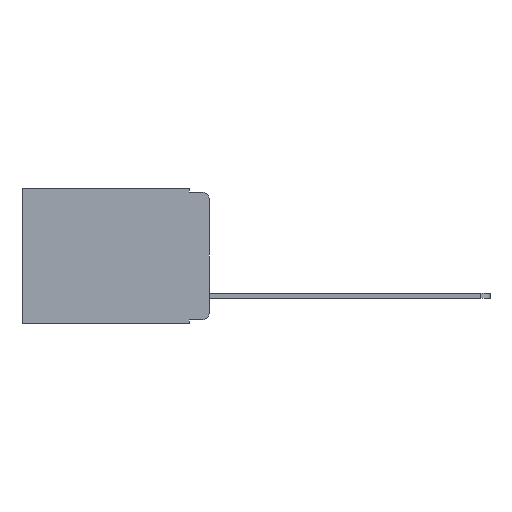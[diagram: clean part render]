
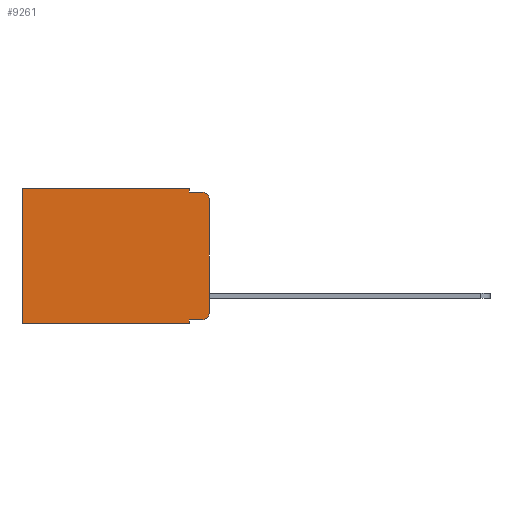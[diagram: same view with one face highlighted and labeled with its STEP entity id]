
A CAD part, left-side view. The second image highlights one B-rep face of the part: STEP entity #9261.
In plain terms, the highlighted planar face has unit normal (-1, 0, 0).
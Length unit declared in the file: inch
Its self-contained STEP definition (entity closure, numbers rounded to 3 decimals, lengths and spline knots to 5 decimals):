
#23 = VERTEX_POINT ( 'NONE', #14910 ) ;
#383 = VERTEX_POINT ( 'NONE', #16294 ) ;
#658 = VERTEX_POINT ( 'NONE', #15442 ) ;
#695 = EDGE_CURVE ( 'NONE', #15312, #2778, #7345, .T. ) ;
#776 = VERTEX_POINT ( 'NONE', #18592 ) ;
#1225 = DIRECTION ( 'NONE',  ( 0., -1., 0. ) ) ;
#1609 = CARTESIAN_POINT ( 'NONE',  ( 0.298, 0., -0.343 ) ) ;
#1758 = PLANE ( 'NONE',  #10505 ) ;
#1880 = EDGE_CURVE ( 'NONE', #15836, #3848, #2449, .T. ) ;
#2449 = LINE ( 'NONE', #13862, #15797 ) ;
#2712 = DIRECTION ( 'NONE',  ( 0., 1., 0. ) ) ;
#2778 = VERTEX_POINT ( 'NONE', #19529 ) ;
#3136 = DIRECTION ( 'NONE',  ( -1., 0., 0. ) ) ;
#3154 = CIRCLE ( 'NONE', #19456, 0.02 ) ;
#3315 = VECTOR ( 'NONE', #5081, 39.37008 ) ;
#3368 = VECTOR ( 'NONE', #15192, 39.37008 ) ;
#3510 = CARTESIAN_POINT ( 'NONE',  ( 0.298, 0., 0. ) ) ;
#3606 = CARTESIAN_POINT ( 'NONE',  ( 0.298, 0.02, -0.03 ) ) ;
#3813 = ORIENTED_EDGE ( 'NONE', *, *, #19001, .F. ) ;
#3848 = VERTEX_POINT ( 'NONE', #4639 ) ;
#3917 = LINE ( 'NONE', #19953, #3368 ) ;
#4080 = ORIENTED_EDGE ( 'NONE', *, *, #5950, .F. ) ;
#4222 = EDGE_CURVE ( 'NONE', #15836, #23, #12175, .T. ) ;
#4639 = CARTESIAN_POINT ( 'NONE',  ( 0.298, 0.02, -0.333 ) ) ;
#4888 = CARTESIAN_POINT ( 'NONE',  ( 0.298, 0.051, 0. ) ) ;
#4897 = CARTESIAN_POINT ( 'NONE',  ( 0.298, 0.051, 0. ) ) ;
#5081 = DIRECTION ( 'NONE',  ( 0., 0., -1. ) ) ;
#5204 = VERTEX_POINT ( 'NONE', #5229 ) ;
#5229 = CARTESIAN_POINT ( 'NONE',  ( 0.298, 0.473, -0.343 ) ) ;
#5275 = DIRECTION ( 'NONE',  ( 1., 0., 0. ) ) ;
#5374 = DIRECTION ( 'NONE',  ( 0., 0., -1. ) ) ;
#5455 = ORIENTED_EDGE ( 'NONE', *, *, #15792, .F. ) ;
#5950 = EDGE_CURVE ( 'NONE', #23, #5204, #6473, .T. ) ;
#5974 = ORIENTED_EDGE ( 'NONE', *, *, #7655, .T. ) ;
#6473 = LINE ( 'NONE', #1609, #18988 ) ;
#6525 = ORIENTED_EDGE ( 'NONE', *, *, #1880, .T. ) ;
#7177 = LINE ( 'NONE', #11380, #18666 ) ;
#7211 = EDGE_LOOP ( 'NONE', ( #5455, #12775, #3813, #7830, #11241, #14544, #4080, #15796, #6525, #5974 ) ) ;
#7345 = LINE ( 'NONE', #4888, #3315 ) ;
#7655 = EDGE_CURVE ( 'NONE', #3848, #383, #3154, .T. ) ;
#7830 = ORIENTED_EDGE ( 'NONE', *, *, #695, .F. ) ;
#8178 = AXIS2_PLACEMENT_3D ( 'NONE', #3606, #15288, #5374 ) ;
#8639 = LINE ( 'NONE', #20809, #16831 ) ;
#9261 = ADVANCED_FACE ( 'NONE', ( #14615 ), #1758, .F. ) ;
#9427 = VERTEX_POINT ( 'NONE', #18761 ) ;
#9924 = VECTOR ( 'NONE', #12578, 39.37008 ) ;
#10505 = AXIS2_PLACEMENT_3D ( 'NONE', #3510, #5275, #16810 ) ;
#11241 = ORIENTED_EDGE ( 'NONE', *, *, #20572, .T. ) ;
#11380 = CARTESIAN_POINT ( 'NONE',  ( 0.298, 0.051, -0.01 ) ) ;
#11689 = VECTOR ( 'NONE', #14607, 39.37008 ) ;
#12029 = CARTESIAN_POINT ( 'NONE',  ( 0.298, 0.051, 0. ) ) ;
#12175 = LINE ( 'NONE', #4897, #11689 ) ;
#12527 = EDGE_CURVE ( 'NONE', #658, #9427, #21482, .T. ) ;
#12578 = DIRECTION ( 'NONE',  ( 0., 0., -1. ) ) ;
#12775 = ORIENTED_EDGE ( 'NONE', *, *, #12527, .T. ) ;
#13237 = CARTESIAN_POINT ( 'NONE',  ( 0.298, 0.02, -0.313 ) ) ;
#13445 = DIRECTION ( 'NONE',  ( 0., 1., 0. ) ) ;
#13862 = CARTESIAN_POINT ( 'NONE',  ( 0.298, 0.051, -0.333 ) ) ;
#14544 = ORIENTED_EDGE ( 'NONE', *, *, #21116, .T. ) ;
#14607 = DIRECTION ( 'NONE',  ( 0., 0., -1. ) ) ;
#14615 = FACE_OUTER_BOUND ( 'NONE', #7211, .T. ) ;
#14846 = DIRECTION ( 'NONE',  ( 0., 0., -1. ) ) ;
#14910 = CARTESIAN_POINT ( 'NONE',  ( 0.298, 0.051, -0.343 ) ) ;
#15192 = DIRECTION ( 'NONE',  ( 0., 0., -1. ) ) ;
#15288 = DIRECTION ( 'NONE',  ( -1., 0., 0. ) ) ;
#15312 = VERTEX_POINT ( 'NONE', #12029 ) ;
#15442 = CARTESIAN_POINT ( 'NONE',  ( 0.298, 0., -0.03 ) ) ;
#15792 = EDGE_CURVE ( 'NONE', #658, #383, #3917, .T. ) ;
#15796 = ORIENTED_EDGE ( 'NONE', *, *, #4222, .F. ) ;
#15797 = VECTOR ( 'NONE', #15970, 39.37008 ) ;
#15836 = VERTEX_POINT ( 'NONE', #20077 ) ;
#15970 = DIRECTION ( 'NONE',  ( 0., -1., 0. ) ) ;
#16294 = CARTESIAN_POINT ( 'NONE',  ( 0.298, 0., -0.313 ) ) ;
#16810 = DIRECTION ( 'NONE',  ( 0., 0., -1. ) ) ;
#16831 = VECTOR ( 'NONE', #2712, 39.37008 ) ;
#18554 = LINE ( 'NONE', #18915, #9924 ) ;
#18592 = CARTESIAN_POINT ( 'NONE',  ( 0.298, 0.473, 0. ) ) ;
#18666 = VECTOR ( 'NONE', #1225, 39.37008 ) ;
#18761 = CARTESIAN_POINT ( 'NONE',  ( 0.298, 0.02, -0.01 ) ) ;
#18915 = CARTESIAN_POINT ( 'NONE',  ( 0.298, 0.473, 0. ) ) ;
#18988 = VECTOR ( 'NONE', #13445, 39.37008 ) ;
#19001 = EDGE_CURVE ( 'NONE', #2778, #9427, #7177, .T. ) ;
#19456 = AXIS2_PLACEMENT_3D ( 'NONE', #13237, #3136, #14846 ) ;
#19529 = CARTESIAN_POINT ( 'NONE',  ( 0.298, 0.051, -0.01 ) ) ;
#19953 = CARTESIAN_POINT ( 'NONE',  ( 0.298, 0., 0. ) ) ;
#20077 = CARTESIAN_POINT ( 'NONE',  ( 0.298, 0.051, -0.333 ) ) ;
#20572 = EDGE_CURVE ( 'NONE', #15312, #776, #8639, .T. ) ;
#20809 = CARTESIAN_POINT ( 'NONE',  ( 0.298, 0., 0. ) ) ;
#21116 = EDGE_CURVE ( 'NONE', #776, #5204, #18554, .T. ) ;
#21482 = CIRCLE ( 'NONE', #8178, 0.02 ) ;
